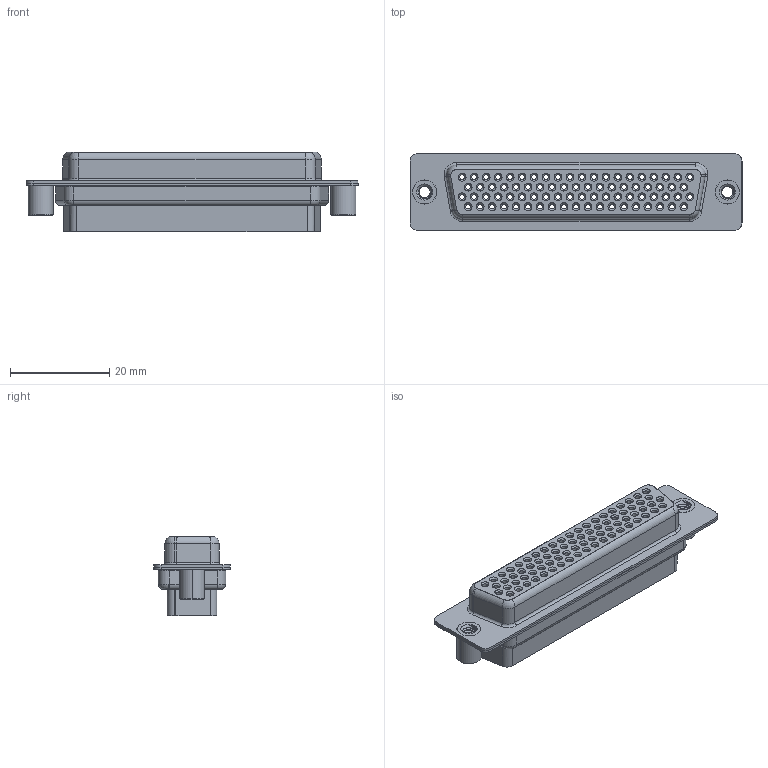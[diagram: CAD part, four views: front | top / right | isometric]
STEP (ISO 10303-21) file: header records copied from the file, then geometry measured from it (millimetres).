
FILE_DESCRIPTION (( 'STEP AP203' ), '1' );
FILE_NAME ('638-078-010-249.STEP', '2020-07-18T16:55:25', ( '' ), ( '' ), 'SwSTEP 2.0', 'SolidWorks 2020', '' );
FILE_SCHEMA (( 'CONFIG_CONTROL_DESIGN' ));
Length unit declared in the file: millimetre
Products named in the file (5): 638-078-010-249; 638 Shell Rear_78 Contacts; 638 4-40 Threaded Standoff BS; 638 Housing_78 Contacts HP; 638 Shell Front_78 Contacts
Assembly tree (5 placements, depth 2):
  638-078-010-249
    638 Housing_78 Contacts HP
    638 Shell Front_78 Contacts
    638 Shell Rear_78 Contacts
    638 4-40 Threaded Standoff BS  x2
Bounding box: 67 x 15.4 x 16.1 mm (x, y, z)
Volume: 6509.2 mm3; surface area: 14901.8 mm2
Topology: 5 solids, 5 shells, 1315 faces, 2933 edges, 1873 vertices
Faces by surface type: cylinder 781, plane 301, cone 170, torus 57, bspline 6
Entity records: 38253 total; most frequent: CARTESIAN_POINT 7806, DIRECTION 6959, ORIENTED_EDGE 5640, AXIS2_PLACEMENT_3D 2960, EDGE_CURVE 2820, VERTEX_POINT 1800, CIRCLE 1684, EDGE_LOOP 1684
